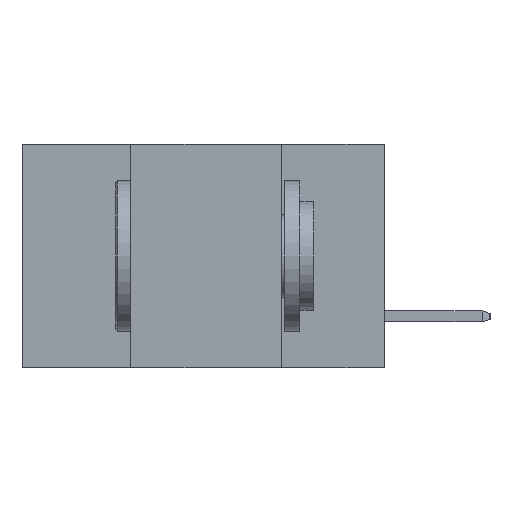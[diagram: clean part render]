
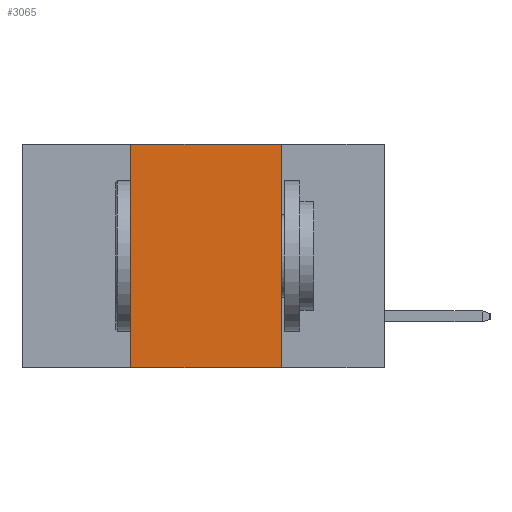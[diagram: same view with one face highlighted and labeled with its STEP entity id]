
A CAD part, left-side view. The second image highlights one B-rep face of the part: STEP entity #3065.
In plain terms, the highlighted planar face has unit normal (-1, 0, 0).
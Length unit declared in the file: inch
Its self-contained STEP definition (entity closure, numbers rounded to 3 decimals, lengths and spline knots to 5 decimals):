
#1212 = VECTOR ( 'NONE', #13519, 39.37008 ) ;
#1480 = VECTOR ( 'NONE', #16595, 39.37008 ) ;
#1621 = LINE ( 'NONE', #4146, #1212 ) ;
#1862 = LINE ( 'NONE', #9873, #15769 ) ;
#3065 = ADVANCED_FACE ( 'NONE', ( #3332 ), #17346, .F. ) ;
#3332 = FACE_OUTER_BOUND ( 'NONE', #15414, .T. ) ;
#3640 = VECTOR ( 'NONE', #14133, 39.37008 ) ;
#3858 = VERTEX_POINT ( 'NONE', #16118 ) ;
#4073 = ORIENTED_EDGE ( 'NONE', *, *, #7062, .F. ) ;
#4146 = CARTESIAN_POINT ( 'NONE',  ( 0., 0.17, 0. ) ) ;
#4761 = CARTESIAN_POINT ( 'NONE',  ( 0., 0.6, 0. ) ) ;
#5073 = CARTESIAN_POINT ( 'NONE',  ( 0., 0.42, 0. ) ) ;
#5942 = CARTESIAN_POINT ( 'NONE',  ( 0., 0.17, 0. ) ) ;
#7062 = EDGE_CURVE ( 'NONE', #7455, #16964, #14375, .T. ) ;
#7172 = EDGE_CURVE ( 'NONE', #3858, #16989, #15413, .T. ) ;
#7455 = VERTEX_POINT ( 'NONE', #5073 ) ;
#7475 = ORIENTED_EDGE ( 'NONE', *, *, #16761, .F. ) ;
#9136 = EDGE_CURVE ( 'NONE', #3858, #7455, #1862, .T. ) ;
#9873 = CARTESIAN_POINT ( 'NONE',  ( 0., 0.42, 0. ) ) ;
#10460 = AXIS2_PLACEMENT_3D ( 'NONE', #16853, #16991, #14784 ) ;
#11187 = ORIENTED_EDGE ( 'NONE', *, *, #9136, .F. ) ;
#13519 = DIRECTION ( 'NONE',  ( 0., 0., -1. ) ) ;
#14133 = DIRECTION ( 'NONE',  ( 0., -1., 0. ) ) ;
#14375 = LINE ( 'NONE', #4761, #3640 ) ;
#14784 = DIRECTION ( 'NONE',  ( 0., 0., -1. ) ) ;
#15348 = CARTESIAN_POINT ( 'NONE',  ( 0., 0.17, -0.37 ) ) ;
#15413 = LINE ( 'NONE', #16691, #1480 ) ;
#15414 = EDGE_LOOP ( 'NONE', ( #7475, #4073, #11187, #16773 ) ) ;
#15769 = VECTOR ( 'NONE', #16498, 39.37008 ) ;
#16118 = CARTESIAN_POINT ( 'NONE',  ( 0., 0.42, -0.37 ) ) ;
#16498 = DIRECTION ( 'NONE',  ( 0., 0., 1. ) ) ;
#16595 = DIRECTION ( 'NONE',  ( 0., -1., 0. ) ) ;
#16691 = CARTESIAN_POINT ( 'NONE',  ( 0., 0.6, -0.37 ) ) ;
#16761 = EDGE_CURVE ( 'NONE', #16964, #16989, #1621, .T. ) ;
#16773 = ORIENTED_EDGE ( 'NONE', *, *, #7172, .T. ) ;
#16853 = CARTESIAN_POINT ( 'NONE',  ( 0., 0.6, 0. ) ) ;
#16964 = VERTEX_POINT ( 'NONE', #5942 ) ;
#16989 = VERTEX_POINT ( 'NONE', #15348 ) ;
#16991 = DIRECTION ( 'NONE',  ( 1., 0., 0. ) ) ;
#17346 = PLANE ( 'NONE',  #10460 ) ;
